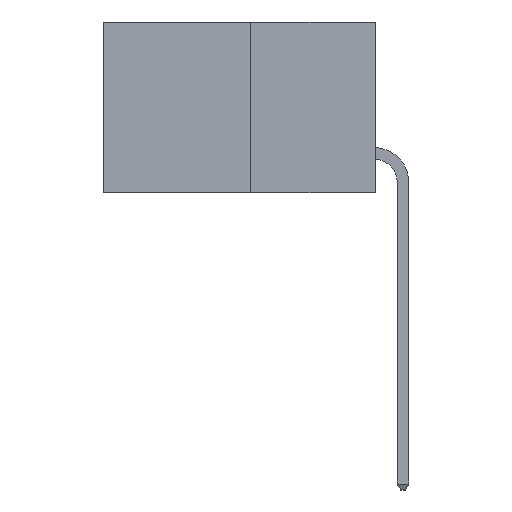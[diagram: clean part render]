
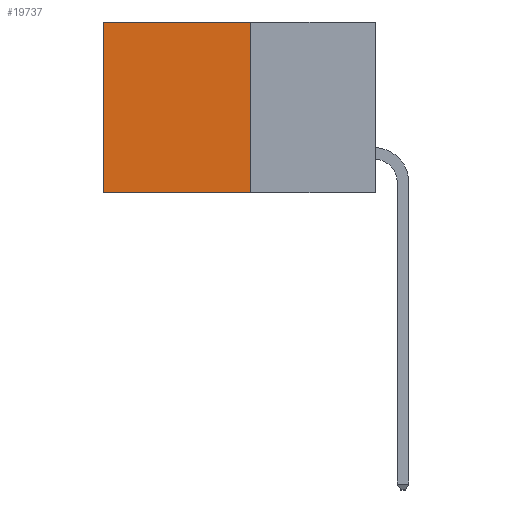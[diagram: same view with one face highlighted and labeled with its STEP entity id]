
A CAD part, left-side view. The second image highlights one B-rep face of the part: STEP entity #19737.
In plain terms, the highlighted planar face has unit normal (-1, 0, 0).
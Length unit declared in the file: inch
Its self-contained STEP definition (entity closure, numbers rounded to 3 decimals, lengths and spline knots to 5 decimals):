
#235 = CARTESIAN_POINT ( 'NONE',  ( 0.277, 0.59, 0. ) ) ;
#519 = ORIENTED_EDGE ( 'NONE', *, *, #13087, .F. ) ;
#612 = CARTESIAN_POINT ( 'NONE',  ( 0.277, 0.59, -0.37 ) ) ;
#1081 = CARTESIAN_POINT ( 'NONE',  ( 0.277, 0.27, 0. ) ) ;
#1584 = VECTOR ( 'NONE', #3561, 39.37008 ) ;
#1591 = ORIENTED_EDGE ( 'NONE', *, *, #7081, .T. ) ;
#1825 = EDGE_CURVE ( 'NONE', #13832, #1958, #1857, .T. ) ;
#1857 = LINE ( 'NONE', #612, #18347 ) ;
#1870 = PLANE ( 'NONE',  #5359 ) ;
#1958 = VERTEX_POINT ( 'NONE', #13350 ) ;
#3551 = DIRECTION ( 'NONE',  ( 1., 0., 0. ) ) ;
#3561 = DIRECTION ( 'NONE',  ( 0., 0., -1. ) ) ;
#3721 = DIRECTION ( 'NONE',  ( 0., 0., -1. ) ) ;
#5359 = AXIS2_PLACEMENT_3D ( 'NONE', #13408, #3551, #15095 ) ;
#5578 = LINE ( 'NONE', #17715, #14308 ) ;
#6071 = LINE ( 'NONE', #15102, #1584 ) ;
#7081 = EDGE_CURVE ( 'NONE', #7935, #13832, #7511, .T. ) ;
#7511 = LINE ( 'NONE', #18393, #19985 ) ;
#7935 = VERTEX_POINT ( 'NONE', #1081 ) ;
#8576 = VERTEX_POINT ( 'NONE', #10593 ) ;
#9864 = ORIENTED_EDGE ( 'NONE', *, *, #1825, .T. ) ;
#10593 = CARTESIAN_POINT ( 'NONE',  ( 0.277, 0.27, -0.37 ) ) ;
#11430 = EDGE_LOOP ( 'NONE', ( #9864, #15768, #519, #1591 ) ) ;
#11636 = EDGE_CURVE ( 'NONE', #8576, #1958, #5578, .T. ) ;
#12697 = FACE_OUTER_BOUND ( 'NONE', #11430, .T. ) ;
#13087 = EDGE_CURVE ( 'NONE', #7935, #8576, #6071, .T. ) ;
#13350 = CARTESIAN_POINT ( 'NONE',  ( 0.277, 0.59, -0.37 ) ) ;
#13408 = CARTESIAN_POINT ( 'NONE',  ( 0.277, 0.27, -0.37 ) ) ;
#13832 = VERTEX_POINT ( 'NONE', #235 ) ;
#14308 = VECTOR ( 'NONE', #20991, 39.37008 ) ;
#15095 = DIRECTION ( 'NONE',  ( 0., 0., -1. ) ) ;
#15102 = CARTESIAN_POINT ( 'NONE',  ( 0.277, 0.27, -0.37 ) ) ;
#15768 = ORIENTED_EDGE ( 'NONE', *, *, #11636, .F. ) ;
#15913 = DIRECTION ( 'NONE',  ( 0., 1., 0. ) ) ;
#17715 = CARTESIAN_POINT ( 'NONE',  ( 0.277, 0.27, -0.37 ) ) ;
#18347 = VECTOR ( 'NONE', #3721, 39.37008 ) ;
#18393 = CARTESIAN_POINT ( 'NONE',  ( 0.277, 0.27, 0. ) ) ;
#19737 = ADVANCED_FACE ( 'NONE', ( #12697 ), #1870, .F. ) ;
#19985 = VECTOR ( 'NONE', #15913, 39.37008 ) ;
#20991 = DIRECTION ( 'NONE',  ( 0., 1., 0. ) ) ;
